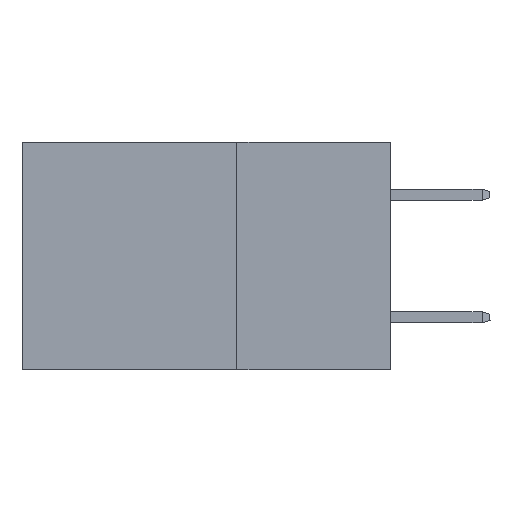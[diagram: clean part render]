
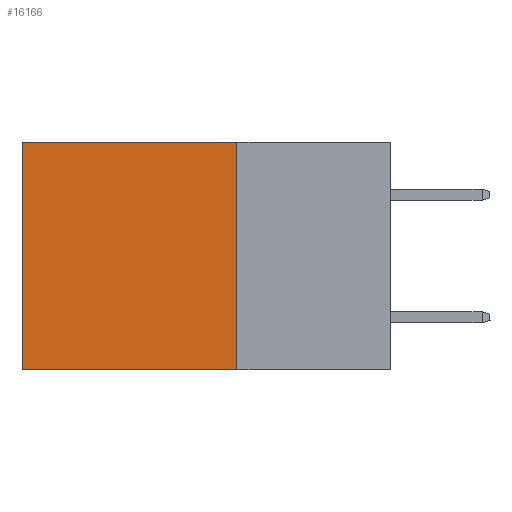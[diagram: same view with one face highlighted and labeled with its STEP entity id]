
A CAD part, left-side view. The second image highlights one B-rep face of the part: STEP entity #16166.
In plain terms, the highlighted planar face has unit normal (-1, 0, 0).
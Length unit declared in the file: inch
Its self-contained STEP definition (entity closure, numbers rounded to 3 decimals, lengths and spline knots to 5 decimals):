
#1612 = CARTESIAN_POINT ( 'NONE',  ( 0.2875, 0.6, 0. ) ) ;
#1823 = CARTESIAN_POINT ( 'NONE',  ( 0.2875, 0.25, 0. ) ) ;
#4063 = VECTOR ( 'NONE', #11139, 39.37008 ) ;
#5801 = VECTOR ( 'NONE', #11380, 39.37008 ) ;
#5932 = VERTEX_POINT ( 'NONE', #14526 ) ;
#6577 = LINE ( 'NONE', #27058, #15219 ) ;
#6945 = LINE ( 'NONE', #21332, #5801 ) ;
#8411 = CARTESIAN_POINT ( 'NONE',  ( 0.2875, 0.25, 0. ) ) ;
#8503 = LINE ( 'NONE', #1612, #26602 ) ;
#10688 = PLANE ( 'NONE',  #28830 ) ;
#10750 = EDGE_CURVE ( 'NONE', #24449, #23571, #22790, .T. ) ;
#11139 = DIRECTION ( 'NONE',  ( 0., 0., -1. ) ) ;
#11380 = DIRECTION ( 'NONE',  ( 0., 1., 0. ) ) ;
#12721 = CARTESIAN_POINT ( 'NONE',  ( 0.2875, 0.6, 0. ) ) ;
#13686 = CARTESIAN_POINT ( 'NONE',  ( 0.2875, 0.25, 0. ) ) ;
#14526 = CARTESIAN_POINT ( 'NONE',  ( 0.2875, 0.6, -0.37 ) ) ;
#15219 = VECTOR ( 'NONE', #15606, 39.37008 ) ;
#15606 = DIRECTION ( 'NONE',  ( 0., 1., 0. ) ) ;
#16166 = ADVANCED_FACE ( 'NONE', ( #29342 ), #10688, .F. ) ;
#17944 = ORIENTED_EDGE ( 'NONE', *, *, #10750, .F. ) ;
#19053 = ORIENTED_EDGE ( 'NONE', *, *, #25297, .T. ) ;
#19535 = ORIENTED_EDGE ( 'NONE', *, *, #23314, .F. ) ;
#20324 = ORIENTED_EDGE ( 'NONE', *, *, #29859, .T. ) ;
#21072 = EDGE_LOOP ( 'NONE', ( #20324, #19535, #17944, #19053 ) ) ;
#21332 = CARTESIAN_POINT ( 'NONE',  ( 0.2875, 0.25, -0.37 ) ) ;
#22580 = DIRECTION ( 'NONE',  ( 0., 0., -1. ) ) ;
#22790 = LINE ( 'NONE', #1823, #4063 ) ;
#23314 = EDGE_CURVE ( 'NONE', #23571, #5932, #6945, .T. ) ;
#23571 = VERTEX_POINT ( 'NONE', #24946 ) ;
#24449 = VERTEX_POINT ( 'NONE', #13686 ) ;
#24766 = DIRECTION ( 'NONE',  ( 1., 0., 0. ) ) ;
#24946 = CARTESIAN_POINT ( 'NONE',  ( 0.2875, 0.25, -0.37 ) ) ;
#25297 = EDGE_CURVE ( 'NONE', #24449, #30125, #6577, .T. ) ;
#26602 = VECTOR ( 'NONE', #22580, 39.37008 ) ;
#27058 = CARTESIAN_POINT ( 'NONE',  ( 0.2875, 0.25, 0. ) ) ;
#27352 = DIRECTION ( 'NONE',  ( 0., 0., -1. ) ) ;
#28830 = AXIS2_PLACEMENT_3D ( 'NONE', #8411, #24766, #27352 ) ;
#29342 = FACE_OUTER_BOUND ( 'NONE', #21072, .T. ) ;
#29859 = EDGE_CURVE ( 'NONE', #30125, #5932, #8503, .T. ) ;
#30125 = VERTEX_POINT ( 'NONE', #12721 ) ;
